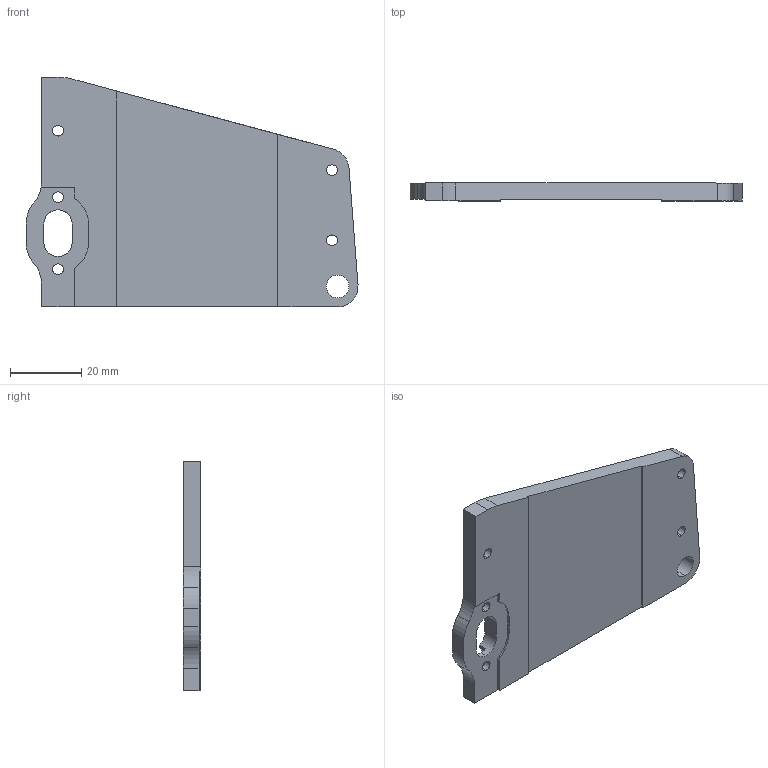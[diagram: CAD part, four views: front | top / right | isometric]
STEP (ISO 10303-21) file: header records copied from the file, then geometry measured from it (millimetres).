
FILE_DESCRIPTION (( 'STEP AP214' ), '1' );
FILE_NAME ('Reinforced_Mag_Well_Right.step', '2015-06-12T17:09:06', ( '' ), ( '' ), 'SwSTEP 2.0', 'SolidWorks 2015', '' );
FILE_SCHEMA (( 'AUTOMOTIVE_DESIGN' ));
Length unit declared in the file: millimetre
Products named in the file (1): Reinforced_Mag_Well_Right
Bounding box: 93 x 5 x 64.36 mm (x, y, z)
Volume: 21623.4 mm3; surface area: 11340.7 mm2
Topology: 1 solids, 1 shells, 81 faces, 228 edges, 152 vertices
Faces by surface type: plane 57, cylinder 24
Entity records: 2677 total; most frequent: CARTESIAN_POINT 462, ORIENTED_EDGE 456, DIRECTION 445, EDGE_CURVE 228, VECTOR 175, LINE 175, VERTEX_POINT 152, AXIS2_PLACEMENT_3D 135
